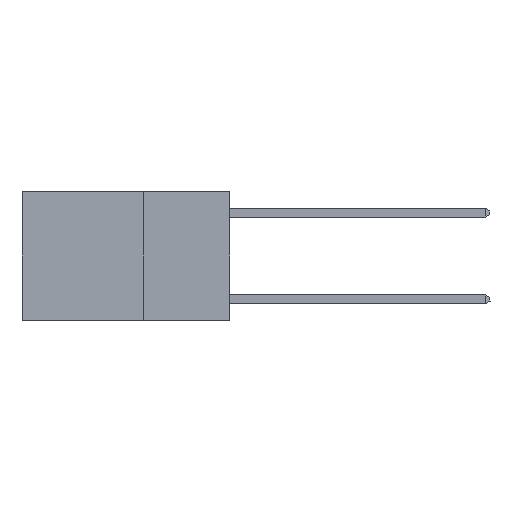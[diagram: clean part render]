
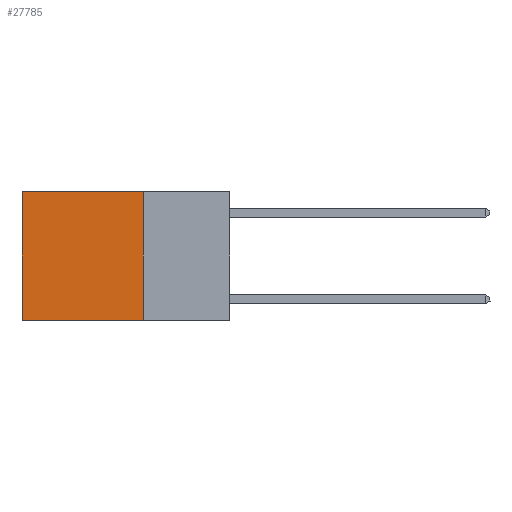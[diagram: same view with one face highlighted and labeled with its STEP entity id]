
A CAD part, left-side view. The second image highlights one B-rep face of the part: STEP entity #27785.
In plain terms, the highlighted planar face has unit normal (-1, 0, 0).
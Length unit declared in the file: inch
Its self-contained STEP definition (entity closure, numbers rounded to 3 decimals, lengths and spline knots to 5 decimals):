
#279 = ORIENTED_EDGE ( 'NONE', *, *, #11140, .T. ) ;
#498 = DIRECTION ( 'NONE',  ( 0., 0., -1. ) ) ;
#1190 = VERTEX_POINT ( 'NONE', #16443 ) ;
#1708 = EDGE_LOOP ( 'NONE', ( #279, #20836, #8156, #28142 ) ) ;
#2363 = CARTESIAN_POINT ( 'NONE',  ( 0.2625, 0.25, -0.37 ) ) ;
#2800 = LINE ( 'NONE', #5520, #3168 ) ;
#3168 = VECTOR ( 'NONE', #9727, 39.37008 ) ;
#3432 = VERTEX_POINT ( 'NONE', #5290 ) ;
#4570 = CARTESIAN_POINT ( 'NONE',  ( 0.2625, 0.25, 0. ) ) ;
#5290 = CARTESIAN_POINT ( 'NONE',  ( 0.2625, 0.25, -0.37 ) ) ;
#5520 = CARTESIAN_POINT ( 'NONE',  ( 0.2625, 0.25, 0. ) ) ;
#6377 = VECTOR ( 'NONE', #18022, 39.37008 ) ;
#6647 = DIRECTION ( 'NONE',  ( 0., 0., -1. ) ) ;
#8156 = ORIENTED_EDGE ( 'NONE', *, *, #14839, .F. ) ;
#9095 = CARTESIAN_POINT ( 'NONE',  ( 0.2625, 0.25, 0. ) ) ;
#9727 = DIRECTION ( 'NONE',  ( 0., 1., 0. ) ) ;
#11061 = LINE ( 'NONE', #9095, #28292 ) ;
#11140 = EDGE_CURVE ( 'NONE', #17135, #1190, #17061, .T. ) ;
#12347 = LINE ( 'NONE', #2363, #6377 ) ;
#13324 = DIRECTION ( 'NONE',  ( 1., 0., 0. ) ) ;
#13426 = DIRECTION ( 'NONE',  ( 0., 0., -1. ) ) ;
#14839 = EDGE_CURVE ( 'NONE', #27284, #3432, #11061, .T. ) ;
#16080 = CARTESIAN_POINT ( 'NONE',  ( 0.2625, 0.6, 0. ) ) ;
#16443 = CARTESIAN_POINT ( 'NONE',  ( 0.2625, 0.6, -0.37 ) ) ;
#16991 = AXIS2_PLACEMENT_3D ( 'NONE', #4570, #13324, #498 ) ;
#17061 = LINE ( 'NONE', #16080, #25487 ) ;
#17135 = VERTEX_POINT ( 'NONE', #25586 ) ;
#17666 = FACE_OUTER_BOUND ( 'NONE', #1708, .T. ) ;
#18022 = DIRECTION ( 'NONE',  ( 0., 1., 0. ) ) ;
#18047 = PLANE ( 'NONE',  #16991 ) ;
#19800 = CARTESIAN_POINT ( 'NONE',  ( 0.2625, 0.25, 0. ) ) ;
#20836 = ORIENTED_EDGE ( 'NONE', *, *, #28185, .F. ) ;
#25487 = VECTOR ( 'NONE', #13426, 39.37008 ) ;
#25586 = CARTESIAN_POINT ( 'NONE',  ( 0.2625, 0.6, 0. ) ) ;
#27284 = VERTEX_POINT ( 'NONE', #19800 ) ;
#27785 = ADVANCED_FACE ( 'NONE', ( #17666 ), #18047, .F. ) ;
#28142 = ORIENTED_EDGE ( 'NONE', *, *, #28367, .T. ) ;
#28185 = EDGE_CURVE ( 'NONE', #3432, #1190, #12347, .T. ) ;
#28292 = VECTOR ( 'NONE', #6647, 39.37008 ) ;
#28367 = EDGE_CURVE ( 'NONE', #27284, #17135, #2800, .T. ) ;
